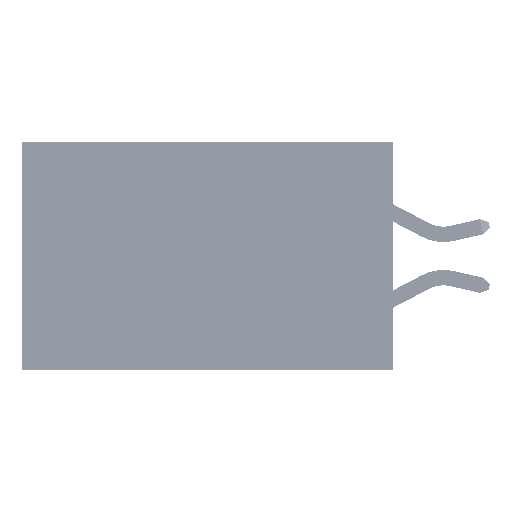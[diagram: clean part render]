
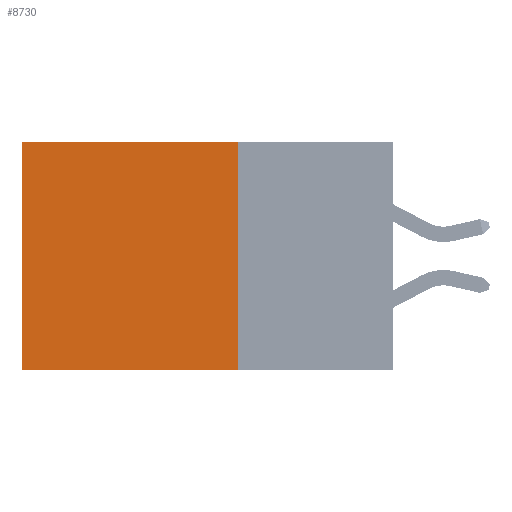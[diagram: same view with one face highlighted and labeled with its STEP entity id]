
A CAD part, left-side view. The second image highlights one B-rep face of the part: STEP entity #8730.
In plain terms, the highlighted planar face has unit normal (-1, 0, 0).
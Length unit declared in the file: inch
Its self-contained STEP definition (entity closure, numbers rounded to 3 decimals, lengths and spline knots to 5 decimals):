
#35 = PLANE ( 'NONE',  #34822 ) ;
#1520 = EDGE_LOOP ( 'NONE', ( #30487, #42278, #42847, #40005 ) ) ;
#3193 = CARTESIAN_POINT ( 'NONE',  ( 0.2875, 0.25, 0. ) ) ;
#3329 = CARTESIAN_POINT ( 'NONE',  ( 0.2875, 0.25, 0. ) ) ;
#7948 = VECTOR ( 'NONE', #44333, 39.37008 ) ;
#8730 = ADVANCED_FACE ( 'NONE', ( #31021 ), #35, .F. ) ;
#10217 = VERTEX_POINT ( 'NONE', #12063 ) ;
#10950 = CARTESIAN_POINT ( 'NONE',  ( 0.2875, 0.25, 0. ) ) ;
#12063 = CARTESIAN_POINT ( 'NONE',  ( 0.2875, 0.25, -0.37 ) ) ;
#12216 = EDGE_CURVE ( 'NONE', #10217, #27028, #38195, .T. ) ;
#14105 = VECTOR ( 'NONE', #17534, 39.37008 ) ;
#16802 = EDGE_CURVE ( 'NONE', #24158, #41169, #35348, .T. ) ;
#17108 = EDGE_CURVE ( 'NONE', #41169, #27028, #37293, .T. ) ;
#17480 = DIRECTION ( 'NONE',  ( 0., 0., -1. ) ) ;
#17534 = DIRECTION ( 'NONE',  ( 0., 1., 0. ) ) ;
#24158 = VERTEX_POINT ( 'NONE', #3329 ) ;
#27028 = VERTEX_POINT ( 'NONE', #33473 ) ;
#27638 = CARTESIAN_POINT ( 'NONE',  ( 0.2875, 0.25, 0. ) ) ;
#29741 = EDGE_CURVE ( 'NONE', #24158, #10217, #44365, .T. ) ;
#29878 = VECTOR ( 'NONE', #30288, 39.37008 ) ;
#30288 = DIRECTION ( 'NONE',  ( 0., 0., -1. ) ) ;
#30487 = ORIENTED_EDGE ( 'NONE', *, *, #17108, .T. ) ;
#30546 = CARTESIAN_POINT ( 'NONE',  ( 0.2875, 0.25, -0.37 ) ) ;
#31021 = FACE_OUTER_BOUND ( 'NONE', #1520, .T. ) ;
#32001 = VECTOR ( 'NONE', #40728, 39.37008 ) ;
#33473 = CARTESIAN_POINT ( 'NONE',  ( 0.2875, 0.6, -0.37 ) ) ;
#34822 = AXIS2_PLACEMENT_3D ( 'NONE', #27638, #41405, #17480 ) ;
#35348 = LINE ( 'NONE', #10950, #14105 ) ;
#37293 = LINE ( 'NONE', #39609, #29878 ) ;
#38195 = LINE ( 'NONE', #30546, #7948 ) ;
#39445 = CARTESIAN_POINT ( 'NONE',  ( 0.2875, 0.6, 0. ) ) ;
#39609 = CARTESIAN_POINT ( 'NONE',  ( 0.2875, 0.6, 0. ) ) ;
#40005 = ORIENTED_EDGE ( 'NONE', *, *, #16802, .T. ) ;
#40728 = DIRECTION ( 'NONE',  ( 0., 0., -1. ) ) ;
#41169 = VERTEX_POINT ( 'NONE', #39445 ) ;
#41405 = DIRECTION ( 'NONE',  ( 1., 0., 0. ) ) ;
#42278 = ORIENTED_EDGE ( 'NONE', *, *, #12216, .F. ) ;
#42847 = ORIENTED_EDGE ( 'NONE', *, *, #29741, .F. ) ;
#44333 = DIRECTION ( 'NONE',  ( 0., 1., 0. ) ) ;
#44365 = LINE ( 'NONE', #3193, #32001 ) ;
